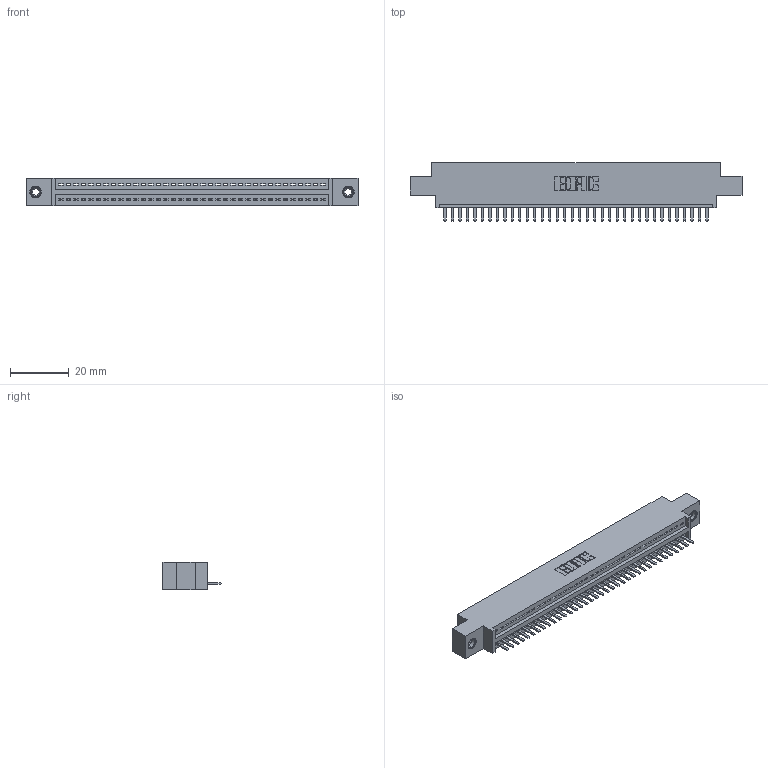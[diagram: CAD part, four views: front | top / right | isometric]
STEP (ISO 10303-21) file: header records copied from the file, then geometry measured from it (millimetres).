
FILE_DESCRIPTION (( 'STEP AP203' ), '1' );
FILE_NAME ('345-036-520-608.STEP', '2019-10-07T22:23:36', ( '' ), ( '' ), 'SwSTEP 2.0', 'SolidWorks 2016', '' );
FILE_SCHEMA (( 'CONFIG_CONTROL_DESIGN' ));
Length unit declared in the file: inch
Products named in the file (4): 345-292-001_345-293-120; 345 Part_0.170 Offset - 0.156 Dia-TI; 345-250-001_345-250-003-102; 345-036-520-608
Assembly tree (39 placements, depth 2):
  345-036-520-608
    345 Part_0.170 Offset - 0.156 Dia-TI
    345-292-001_345-293-120  x36
    345-250-001_345-250-003-102  x2
Bounding box: 112.65 x 19.68 x 9.4 mm (x, y, z)
Volume: 10426.9 mm3; surface area: 13581.8 mm2
Topology: 39 solids, 39 shells, 2422 faces, 7113 edges, 4638 vertices
Faces by surface type: plane 1628, cylinder 778, cone 12, torus 4
Entity records: 29334 total; most frequent: CARTESIAN_POINT 5075, ORIENTED_EDGE 5026, DIRECTION 4455, EDGE_CURVE 2513, VECTOR 2213, LINE 2213, VERTEX_POINT 1668, AXIS2_PLACEMENT_3D 1121
